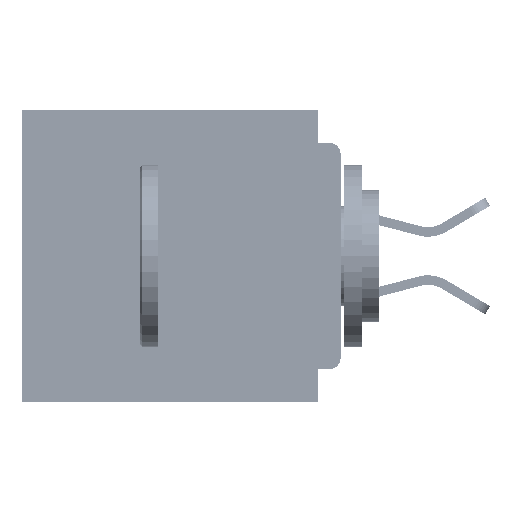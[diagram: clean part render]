
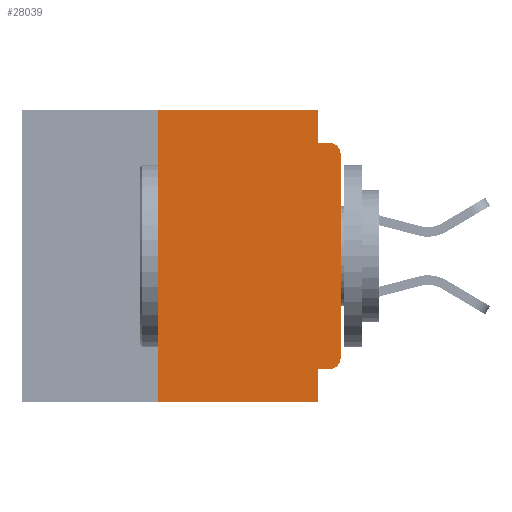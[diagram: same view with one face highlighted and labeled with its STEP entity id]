
A CAD part, left-side view. The second image highlights one B-rep face of the part: STEP entity #28039.
In plain terms, the highlighted planar face has unit normal (-1, 0, 0).
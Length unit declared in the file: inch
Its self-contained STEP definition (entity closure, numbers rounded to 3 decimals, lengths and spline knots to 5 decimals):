
#827 = EDGE_CURVE ( 'NONE', #39909, #25805, #45116, .T. ) ;
#1469 = LINE ( 'NONE', #52676, #28003 ) ;
#1557 = VECTOR ( 'NONE', #3397, 39.37008 ) ;
#2741 = DIRECTION ( 'NONE',  ( 0., 0., 1. ) ) ;
#3397 = DIRECTION ( 'NONE',  ( 0., 1., 0. ) ) ;
#4163 = DIRECTION ( 'NONE',  ( 0., 0., -1. ) ) ;
#4274 = CARTESIAN_POINT ( 'NONE',  ( 0., 0.015, -0.045 ) ) ;
#4422 = CARTESIAN_POINT ( 'NONE',  ( 0., 0.031, -0.045 ) ) ;
#5164 = CARTESIAN_POINT ( 'NONE',  ( 0., 0., -0.06 ) ) ;
#5834 = EDGE_CURVE ( 'NONE', #56496, #24489, #1469, .T. ) ;
#6529 = VECTOR ( 'NONE', #34448, 39.37008 ) ;
#6606 = EDGE_CURVE ( 'NONE', #56216, #56496, #43131, .T. ) ;
#8094 = CARTESIAN_POINT ( 'NONE',  ( 0., 0.25, -0.4 ) ) ;
#8473 = VECTOR ( 'NONE', #10403, 39.37008 ) ;
#9125 = ORIENTED_EDGE ( 'NONE', *, *, #42961, .F. ) ;
#10282 = ORIENTED_EDGE ( 'NONE', *, *, #20458, .T. ) ;
#10403 = DIRECTION ( 'NONE',  ( 0., 0., -1. ) ) ;
#12499 = CARTESIAN_POINT ( 'NONE',  ( 0., 0.015, -0.355 ) ) ;
#12631 = CARTESIAN_POINT ( 'NONE',  ( 0., 0.015, -0.06 ) ) ;
#12789 = AXIS2_PLACEMENT_3D ( 'NONE', #12631, #49601, #17994 ) ;
#13154 = ORIENTED_EDGE ( 'NONE', *, *, #47262, .T. ) ;
#13472 = ORIENTED_EDGE ( 'NONE', *, *, #6606, .F. ) ;
#14588 = PLANE ( 'NONE',  #33230 ) ;
#14734 = EDGE_CURVE ( 'NONE', #24489, #23870, #19368, .T. ) ;
#15687 = LINE ( 'NONE', #61389, #1557 ) ;
#15726 = ORIENTED_EDGE ( 'NONE', *, *, #44078, .T. ) ;
#16846 = ORIENTED_EDGE ( 'NONE', *, *, #38911, .F. ) ;
#16994 = ORIENTED_EDGE ( 'NONE', *, *, #5834, .F. ) ;
#17265 = CARTESIAN_POINT ( 'NONE',  ( 0., 0., -0.045 ) ) ;
#17994 = DIRECTION ( 'NONE',  ( 0., 0., -1. ) ) ;
#19368 = LINE ( 'NONE', #17265, #64803 ) ;
#19930 = CARTESIAN_POINT ( 'NONE',  ( 0., 0.437, 0. ) ) ;
#20458 = EDGE_CURVE ( 'NONE', #59784, #39909, #55101, .T. ) ;
#20656 = LINE ( 'NONE', #8094, #6529 ) ;
#20745 = CARTESIAN_POINT ( 'NONE',  ( 0., 0.437, -0.4 ) ) ;
#21390 = DIRECTION ( 'NONE',  ( -1., 0., 0. ) ) ;
#22638 = CARTESIAN_POINT ( 'NONE',  ( 0., 0.25, -0.4 ) ) ;
#23870 = VERTEX_POINT ( 'NONE', #4274 ) ;
#24222 = LINE ( 'NONE', #47380, #8473 ) ;
#24489 = VERTEX_POINT ( 'NONE', #4422 ) ;
#25131 = DIRECTION ( 'NONE',  ( 0., -1., 0. ) ) ;
#25805 = VERTEX_POINT ( 'NONE', #5164 ) ;
#28003 = VECTOR ( 'NONE', #47576, 39.37008 ) ;
#28039 = ADVANCED_FACE ( 'NONE', ( #67432 ), #14588, .F. ) ;
#28369 = CARTESIAN_POINT ( 'NONE',  ( 0., 0.25, 0. ) ) ;
#32421 = VERTEX_POINT ( 'NONE', #42425 ) ;
#33230 = AXIS2_PLACEMENT_3D ( 'NONE', #19930, #35835, #4163 ) ;
#34407 = CARTESIAN_POINT ( 'NONE',  ( 0., 0., 0. ) ) ;
#34448 = DIRECTION ( 'NONE',  ( 0., 0., 1. ) ) ;
#35638 = VECTOR ( 'NONE', #63005, 39.37008 ) ;
#35835 = DIRECTION ( 'NONE',  ( 1., 0., 0. ) ) ;
#35974 = CARTESIAN_POINT ( 'NONE',  ( 0., 0.031, 0. ) ) ;
#37736 = VERTEX_POINT ( 'NONE', #38214 ) ;
#38214 = CARTESIAN_POINT ( 'NONE',  ( 0., 0.031, -0.355 ) ) ;
#38308 = ORIENTED_EDGE ( 'NONE', *, *, #14734, .F. ) ;
#38911 = EDGE_CURVE ( 'NONE', #59784, #37736, #15687, .T. ) ;
#39014 = ORIENTED_EDGE ( 'NONE', *, *, #51881, .F. ) ;
#39909 = VERTEX_POINT ( 'NONE', #53862 ) ;
#41483 = VECTOR ( 'NONE', #25131, 39.37008 ) ;
#41934 = AXIS2_PLACEMENT_3D ( 'NONE', #52988, #21390, #58315 ) ;
#42425 = CARTESIAN_POINT ( 'NONE',  ( 0., 0.031, -0.4 ) ) ;
#42961 = EDGE_CURVE ( 'NONE', #37736, #32421, #24222, .T. ) ;
#43131 = LINE ( 'NONE', #67366, #41483 ) ;
#44078 = EDGE_CURVE ( 'NONE', #52391, #32421, #51319, .T. ) ;
#45116 = LINE ( 'NONE', #34407, #59165 ) ;
#47262 = EDGE_CURVE ( 'NONE', #25805, #23870, #62561, .T. ) ;
#47380 = CARTESIAN_POINT ( 'NONE',  ( 0., 0.031, -0.4 ) ) ;
#47576 = DIRECTION ( 'NONE',  ( 0., 0., -1. ) ) ;
#47902 = EDGE_LOOP ( 'NONE', ( #50179, #13154, #38308, #16994, #13472, #39014, #15726, #9125, #16846, #10282 ) ) ;
#49601 = DIRECTION ( 'NONE',  ( -1., 0., 0. ) ) ;
#50179 = ORIENTED_EDGE ( 'NONE', *, *, #827, .T. ) ;
#51319 = LINE ( 'NONE', #20745, #35638 ) ;
#51881 = EDGE_CURVE ( 'NONE', #52391, #56216, #20656, .T. ) ;
#52391 = VERTEX_POINT ( 'NONE', #22638 ) ;
#52676 = CARTESIAN_POINT ( 'NONE',  ( 0., 0.031, 0. ) ) ;
#52988 = CARTESIAN_POINT ( 'NONE',  ( 0., 0.015, -0.34 ) ) ;
#53862 = CARTESIAN_POINT ( 'NONE',  ( 0., 0., -0.34 ) ) ;
#54189 = DIRECTION ( 'NONE',  ( 0., -1., 0. ) ) ;
#55101 = CIRCLE ( 'NONE', #41934, 0.015 ) ;
#56216 = VERTEX_POINT ( 'NONE', #28369 ) ;
#56496 = VERTEX_POINT ( 'NONE', #35974 ) ;
#58315 = DIRECTION ( 'NONE',  ( 0., 0., -1. ) ) ;
#59165 = VECTOR ( 'NONE', #2741, 39.37008 ) ;
#59784 = VERTEX_POINT ( 'NONE', #12499 ) ;
#61389 = CARTESIAN_POINT ( 'NONE',  ( 0., 0., -0.355 ) ) ;
#62561 = CIRCLE ( 'NONE', #12789, 0.015 ) ;
#63005 = DIRECTION ( 'NONE',  ( 0., -1., 0. ) ) ;
#64803 = VECTOR ( 'NONE', #54189, 39.37008 ) ;
#67366 = CARTESIAN_POINT ( 'NONE',  ( 0., 0.437, 0. ) ) ;
#67432 = FACE_OUTER_BOUND ( 'NONE', #47902, .T. ) ;
